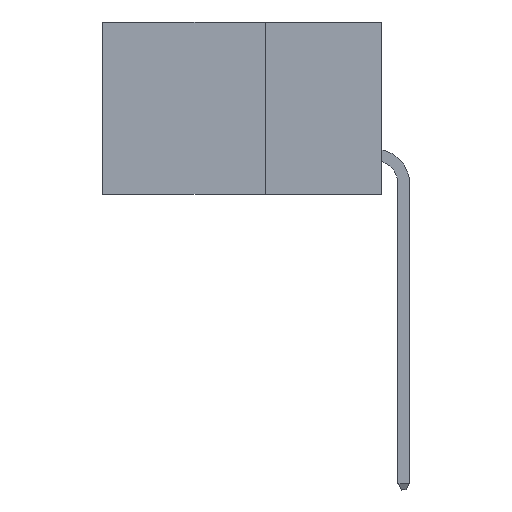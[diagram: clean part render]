
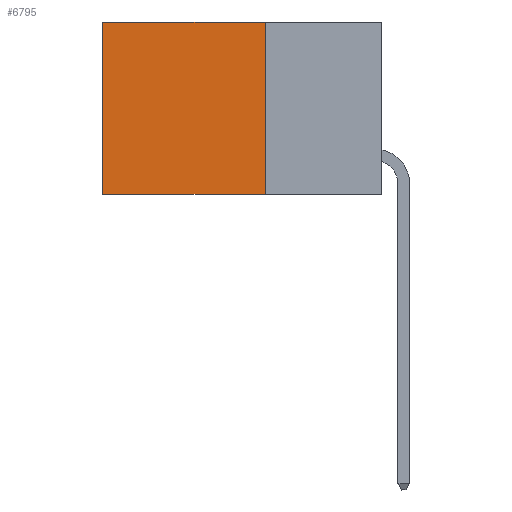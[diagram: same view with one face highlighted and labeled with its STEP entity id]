
A CAD part, left-side view. The second image highlights one B-rep face of the part: STEP entity #6795.
In plain terms, the highlighted planar face has unit normal (-1, 0, 0).
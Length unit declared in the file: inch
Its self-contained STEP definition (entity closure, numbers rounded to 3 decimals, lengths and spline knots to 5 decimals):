
#549 = LINE ( 'NONE', #5803, #5392 ) ;
#959 = DIRECTION ( 'NONE',  ( 0., 0., -1. ) ) ;
#1021 = VERTEX_POINT ( 'NONE', #6757 ) ;
#1360 = CARTESIAN_POINT ( 'NONE',  ( 0.2875, 0.25, -0.37 ) ) ;
#1700 = CARTESIAN_POINT ( 'NONE',  ( 0.2875, 0.25, -0.37 ) ) ;
#2747 = DIRECTION ( 'NONE',  ( 0., 0., -1. ) ) ;
#3538 = VECTOR ( 'NONE', #8202, 39.37008 ) ;
#3557 = EDGE_CURVE ( 'NONE', #5903, #1021, #9247, .T. ) ;
#3690 = EDGE_CURVE ( 'NONE', #7520, #1021, #6095, .T. ) ;
#4538 = VERTEX_POINT ( 'NONE', #7280 ) ;
#4642 = AXIS2_PLACEMENT_3D ( 'NONE', #11762, #10779, #10899 ) ;
#4683 = ORIENTED_EDGE ( 'NONE', *, *, #9009, .F. ) ;
#4839 = VECTOR ( 'NONE', #5209, 39.37008 ) ;
#5209 = DIRECTION ( 'NONE',  ( 0., 1., 0. ) ) ;
#5392 = VECTOR ( 'NONE', #959, 39.37008 ) ;
#5656 = EDGE_CURVE ( 'NONE', #4538, #5903, #6631, .T. ) ;
#5803 = CARTESIAN_POINT ( 'NONE',  ( 0.2875, 0.25, 0. ) ) ;
#5903 = VERTEX_POINT ( 'NONE', #6154 ) ;
#6095 = LINE ( 'NONE', #1360, #3538 ) ;
#6154 = CARTESIAN_POINT ( 'NONE',  ( 0.2875, 0.6, 0. ) ) ;
#6394 = VECTOR ( 'NONE', #2747, 39.37008 ) ;
#6631 = LINE ( 'NONE', #10976, #4839 ) ;
#6757 = CARTESIAN_POINT ( 'NONE',  ( 0.2875, 0.6, -0.37 ) ) ;
#6795 = ADVANCED_FACE ( 'NONE', ( #10235 ), #8834, .F. ) ;
#7280 = CARTESIAN_POINT ( 'NONE',  ( 0.2875, 0.25, 0. ) ) ;
#7520 = VERTEX_POINT ( 'NONE', #1700 ) ;
#8134 = ORIENTED_EDGE ( 'NONE', *, *, #3690, .F. ) ;
#8202 = DIRECTION ( 'NONE',  ( 0., 1., 0. ) ) ;
#8834 = PLANE ( 'NONE',  #4642 ) ;
#9009 = EDGE_CURVE ( 'NONE', #4538, #7520, #549, .T. ) ;
#9240 = EDGE_LOOP ( 'NONE', ( #10443, #8134, #4683, #12075 ) ) ;
#9247 = LINE ( 'NONE', #12025, #6394 ) ;
#10235 = FACE_OUTER_BOUND ( 'NONE', #9240, .T. ) ;
#10443 = ORIENTED_EDGE ( 'NONE', *, *, #3557, .T. ) ;
#10779 = DIRECTION ( 'NONE',  ( 1., 0., 0. ) ) ;
#10899 = DIRECTION ( 'NONE',  ( 0., 0., -1. ) ) ;
#10976 = CARTESIAN_POINT ( 'NONE',  ( 0.2875, 0.25, 0. ) ) ;
#11762 = CARTESIAN_POINT ( 'NONE',  ( 0.2875, 0.25, 0. ) ) ;
#12025 = CARTESIAN_POINT ( 'NONE',  ( 0.2875, 0.6, 0. ) ) ;
#12075 = ORIENTED_EDGE ( 'NONE', *, *, #5656, .T. ) ;
